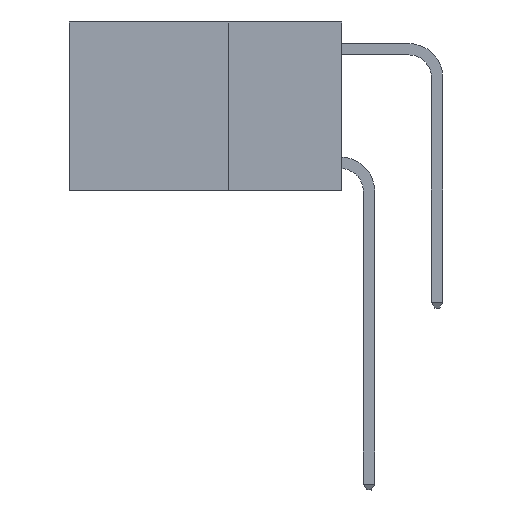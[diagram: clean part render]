
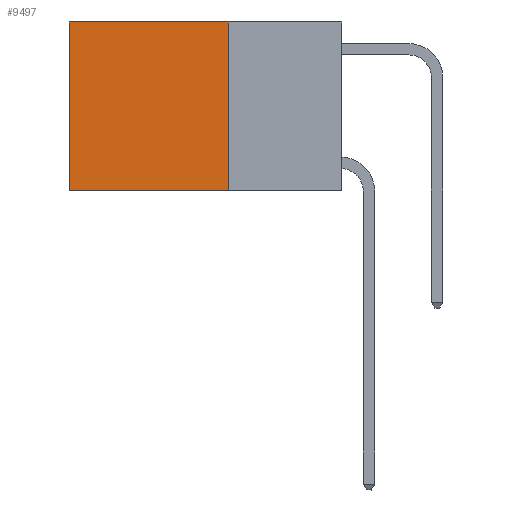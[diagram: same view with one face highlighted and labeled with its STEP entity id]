
A CAD part, left-side view. The second image highlights one B-rep face of the part: STEP entity #9497.
In plain terms, the highlighted planar face has unit normal (-1, 0, 0).
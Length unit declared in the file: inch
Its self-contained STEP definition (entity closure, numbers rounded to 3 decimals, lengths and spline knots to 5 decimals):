
#241 = DIRECTION ( 'NONE',  ( 0., 0., -1. ) ) ;
#424 = DIRECTION ( 'NONE',  ( 0., 1., 0. ) ) ;
#891 = DIRECTION ( 'NONE',  ( 1., 0., 0. ) ) ;
#1756 = CARTESIAN_POINT ( 'NONE',  ( 0.2625, 0.6, -0.37 ) ) ;
#2513 = VECTOR ( 'NONE', #15997, 39.37008 ) ;
#2607 = CARTESIAN_POINT ( 'NONE',  ( 0.2625, 0.25, 0. ) ) ;
#2879 = VERTEX_POINT ( 'NONE', #1756 ) ;
#2941 = LINE ( 'NONE', #7776, #2513 ) ;
#3468 = FACE_OUTER_BOUND ( 'NONE', #14388, .T. ) ;
#4633 = VECTOR ( 'NONE', #424, 39.37008 ) ;
#5275 = VERTEX_POINT ( 'NONE', #15797 ) ;
#5512 = CARTESIAN_POINT ( 'NONE',  ( 0.2625, 0.25, 0. ) ) ;
#5603 = VERTEX_POINT ( 'NONE', #5512 ) ;
#6675 = EDGE_CURVE ( 'NONE', #5275, #2879, #8314, .T. ) ;
#7297 = ORIENTED_EDGE ( 'NONE', *, *, #17151, .T. ) ;
#7419 = CARTESIAN_POINT ( 'NONE',  ( 0.2625, 0.25, -0.37 ) ) ;
#7776 = CARTESIAN_POINT ( 'NONE',  ( 0.2625, 0.25, 0. ) ) ;
#8314 = LINE ( 'NONE', #7419, #4633 ) ;
#8798 = LINE ( 'NONE', #10030, #16081 ) ;
#9497 = ADVANCED_FACE ( 'NONE', ( #3468 ), #16086, .F. ) ;
#10025 = VERTEX_POINT ( 'NONE', #17267 ) ;
#10030 = CARTESIAN_POINT ( 'NONE',  ( 0.2625, 0.6, 0. ) ) ;
#10627 = DIRECTION ( 'NONE',  ( 0., 0., -1. ) ) ;
#10983 = EDGE_CURVE ( 'NONE', #5603, #5275, #12239, .T. ) ;
#11283 = ORIENTED_EDGE ( 'NONE', *, *, #6675, .F. ) ;
#11687 = AXIS2_PLACEMENT_3D ( 'NONE', #17471, #891, #10627 ) ;
#12012 = EDGE_CURVE ( 'NONE', #10025, #2879, #8798, .T. ) ;
#12239 = LINE ( 'NONE', #2607, #15478 ) ;
#13280 = ORIENTED_EDGE ( 'NONE', *, *, #12012, .T. ) ;
#13639 = DIRECTION ( 'NONE',  ( 0., 0., -1. ) ) ;
#14388 = EDGE_LOOP ( 'NONE', ( #13280, #11283, #16036, #7297 ) ) ;
#15478 = VECTOR ( 'NONE', #13639, 39.37008 ) ;
#15797 = CARTESIAN_POINT ( 'NONE',  ( 0.2625, 0.25, -0.37 ) ) ;
#15997 = DIRECTION ( 'NONE',  ( 0., 1., 0. ) ) ;
#16036 = ORIENTED_EDGE ( 'NONE', *, *, #10983, .F. ) ;
#16081 = VECTOR ( 'NONE', #241, 39.37008 ) ;
#16086 = PLANE ( 'NONE',  #11687 ) ;
#17151 = EDGE_CURVE ( 'NONE', #5603, #10025, #2941, .T. ) ;
#17267 = CARTESIAN_POINT ( 'NONE',  ( 0.2625, 0.6, 0. ) ) ;
#17471 = CARTESIAN_POINT ( 'NONE',  ( 0.2625, 0.25, 0. ) ) ;
